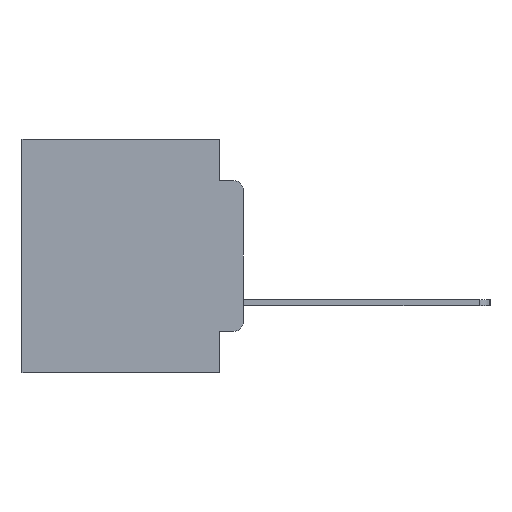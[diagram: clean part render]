
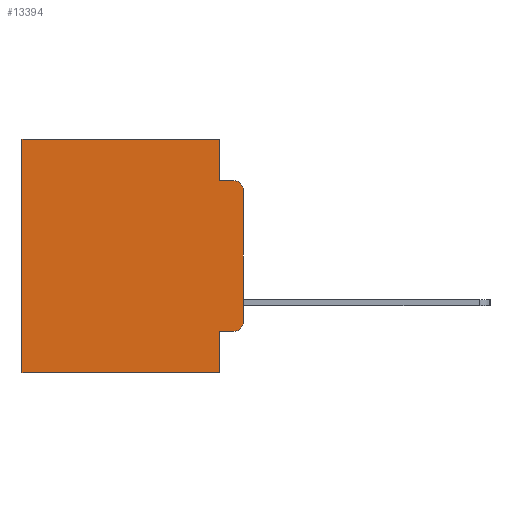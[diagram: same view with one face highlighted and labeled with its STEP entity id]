
A CAD part, left-side view. The second image highlights one B-rep face of the part: STEP entity #13394.
In plain terms, the highlighted planar face has unit normal (-1, 0, 0).
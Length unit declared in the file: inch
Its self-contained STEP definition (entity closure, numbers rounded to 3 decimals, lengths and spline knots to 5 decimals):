
#56 = DIRECTION ( 'NONE',  ( 0., 0., -1. ) ) ;
#273 = VECTOR ( 'NONE', #4384, 39.37008 ) ;
#530 = ORIENTED_EDGE ( 'NONE', *, *, #6574, .T. ) ;
#1505 = ORIENTED_EDGE ( 'NONE', *, *, #19453, .F. ) ;
#2241 = CARTESIAN_POINT ( 'NONE',  ( 0.298, 0.051, 0. ) ) ;
#2369 = VERTEX_POINT ( 'NONE', #10803 ) ;
#2629 = LINE ( 'NONE', #2241, #16949 ) ;
#3151 = EDGE_CURVE ( 'NONE', #2369, #9970, #5638, .T. ) ;
#3416 = ORIENTED_EDGE ( 'NONE', *, *, #10349, .F. ) ;
#3620 = CARTESIAN_POINT ( 'NONE',  ( 0.298, 0.051, -0.5 ) ) ;
#4009 = VECTOR ( 'NONE', #4537, 39.37008 ) ;
#4271 = DIRECTION ( 'NONE',  ( 0., 0., -1. ) ) ;
#4384 = DIRECTION ( 'NONE',  ( 0., 1., 0. ) ) ;
#4537 = DIRECTION ( 'NONE',  ( 0., 0., -1. ) ) ;
#5165 = EDGE_CURVE ( 'NONE', #20581, #14023, #22735, .T. ) ;
#5210 = CARTESIAN_POINT ( 'NONE',  ( 0.298, 0.473, 0. ) ) ;
#5472 = LINE ( 'NONE', #23389, #14577 ) ;
#5638 = CIRCLE ( 'NONE', #23955, 0.02 ) ;
#5688 = LINE ( 'NONE', #10076, #273 ) ;
#5811 = CARTESIAN_POINT ( 'NONE',  ( 0.298, 0.051, -0.4115 ) ) ;
#5874 = CARTESIAN_POINT ( 'NONE',  ( 0.298, 0., 0. ) ) ;
#6372 = CARTESIAN_POINT ( 'NONE',  ( 0.298, 0.02, -0.1085 ) ) ;
#6375 = CARTESIAN_POINT ( 'NONE',  ( 0.298, 0., -0.3915 ) ) ;
#6574 = EDGE_CURVE ( 'NONE', #22520, #19574, #9863, .T. ) ;
#7232 = VECTOR ( 'NONE', #12641, 39.37008 ) ;
#7576 = CARTESIAN_POINT ( 'NONE',  ( 0.298, 0.051, -0.4115 ) ) ;
#7767 = DIRECTION ( 'NONE',  ( 1., 0., 0. ) ) ;
#8082 = VECTOR ( 'NONE', #19365, 39.37008 ) ;
#8307 = ORIENTED_EDGE ( 'NONE', *, *, #21490, .F. ) ;
#9863 = LINE ( 'NONE', #24904, #19579 ) ;
#9929 = CARTESIAN_POINT ( 'NONE',  ( 0.298, 0.051, 0. ) ) ;
#9970 = VERTEX_POINT ( 'NONE', #6375 ) ;
#10076 = CARTESIAN_POINT ( 'NONE',  ( 0.298, 0., -0.5 ) ) ;
#10349 = EDGE_CURVE ( 'NONE', #22870, #22861, #2629, .T. ) ;
#10803 = CARTESIAN_POINT ( 'NONE',  ( 0.298, 0.02, -0.4115 ) ) ;
#10971 = EDGE_CURVE ( 'NONE', #19255, #2369, #23442, .T. ) ;
#11930 = ORIENTED_EDGE ( 'NONE', *, *, #5165, .T. ) ;
#12320 = DIRECTION ( 'NONE',  ( 0., 1., 0. ) ) ;
#12373 = LINE ( 'NONE', #14451, #7232 ) ;
#12451 = FACE_OUTER_BOUND ( 'NONE', #15880, .T. ) ;
#12641 = DIRECTION ( 'NONE',  ( 0., -1., 0. ) ) ;
#12644 = VECTOR ( 'NONE', #12320, 39.37008 ) ;
#12740 = CARTESIAN_POINT ( 'NONE',  ( 0.298, 0.473, -0.5 ) ) ;
#13394 = ADVANCED_FACE ( 'NONE', ( #12451 ), #17462, .F. ) ;
#14023 = VERTEX_POINT ( 'NONE', #14732 ) ;
#14103 = ORIENTED_EDGE ( 'NONE', *, *, #3151, .T. ) ;
#14294 = CARTESIAN_POINT ( 'NONE',  ( 0.298, 0., 0. ) ) ;
#14451 = CARTESIAN_POINT ( 'NONE',  ( 0.298, 0.051, -0.0885 ) ) ;
#14577 = VECTOR ( 'NONE', #56, 39.37008 ) ;
#14732 = CARTESIAN_POINT ( 'NONE',  ( 0.298, 0.02, -0.0885 ) ) ;
#14934 = EDGE_CURVE ( 'NONE', #22870, #22520, #22858, .T. ) ;
#15880 = EDGE_LOOP ( 'NONE', ( #1505, #11930, #22768, #3416, #25106, #530, #18042, #8307, #18660, #14103 ) ) ;
#16183 = CARTESIAN_POINT ( 'NONE',  ( 0.298, 0., 0. ) ) ;
#16949 = VECTOR ( 'NONE', #4271, 39.37008 ) ;
#17375 = DIRECTION ( 'NONE',  ( 0., 0., -1. ) ) ;
#17462 = PLANE ( 'NONE',  #24114 ) ;
#18042 = ORIENTED_EDGE ( 'NONE', *, *, #22515, .F. ) ;
#18660 = ORIENTED_EDGE ( 'NONE', *, *, #10971, .T. ) ;
#19255 = VERTEX_POINT ( 'NONE', #7576 ) ;
#19365 = DIRECTION ( 'NONE',  ( 0., -1., 0. ) ) ;
#19453 = EDGE_CURVE ( 'NONE', #20581, #9970, #24484, .T. ) ;
#19574 = VERTEX_POINT ( 'NONE', #12740 ) ;
#19579 = VECTOR ( 'NONE', #17375, 39.37008 ) ;
#20329 = DIRECTION ( 'NONE',  ( -1., 0., 0. ) ) ;
#20399 = DIRECTION ( 'NONE',  ( -1., 0., 0. ) ) ;
#20404 = CARTESIAN_POINT ( 'NONE',  ( 0.298, 0.02, -0.3915 ) ) ;
#20581 = VERTEX_POINT ( 'NONE', #21308 ) ;
#20792 = DIRECTION ( 'NONE',  ( 0., 0., -1. ) ) ;
#21308 = CARTESIAN_POINT ( 'NONE',  ( 0.298, 0., -0.1085 ) ) ;
#21309 = DIRECTION ( 'NONE',  ( 0., 0., -1. ) ) ;
#21490 = EDGE_CURVE ( 'NONE', #19255, #22686, #5472, .T. ) ;
#22379 = EDGE_CURVE ( 'NONE', #22861, #14023, #12373, .T. ) ;
#22515 = EDGE_CURVE ( 'NONE', #22686, #19574, #5688, .T. ) ;
#22520 = VERTEX_POINT ( 'NONE', #5210 ) ;
#22632 = DIRECTION ( 'NONE',  ( 0., 0., -1. ) ) ;
#22686 = VERTEX_POINT ( 'NONE', #3620 ) ;
#22735 = CIRCLE ( 'NONE', #24955, 0.02 ) ;
#22768 = ORIENTED_EDGE ( 'NONE', *, *, #22379, .F. ) ;
#22858 = LINE ( 'NONE', #14294, #12644 ) ;
#22861 = VERTEX_POINT ( 'NONE', #23335 ) ;
#22870 = VERTEX_POINT ( 'NONE', #9929 ) ;
#23335 = CARTESIAN_POINT ( 'NONE',  ( 0.298, 0.051, -0.0885 ) ) ;
#23389 = CARTESIAN_POINT ( 'NONE',  ( 0.298, 0.051, 0. ) ) ;
#23442 = LINE ( 'NONE', #5811, #8082 ) ;
#23955 = AXIS2_PLACEMENT_3D ( 'NONE', #20404, #20329, #20792 ) ;
#24114 = AXIS2_PLACEMENT_3D ( 'NONE', #5874, #7767, #21309 ) ;
#24484 = LINE ( 'NONE', #16183, #4009 ) ;
#24904 = CARTESIAN_POINT ( 'NONE',  ( 0.298, 0.473, 0. ) ) ;
#24955 = AXIS2_PLACEMENT_3D ( 'NONE', #6372, #20399, #22632 ) ;
#25106 = ORIENTED_EDGE ( 'NONE', *, *, #14934, .T. ) ;
